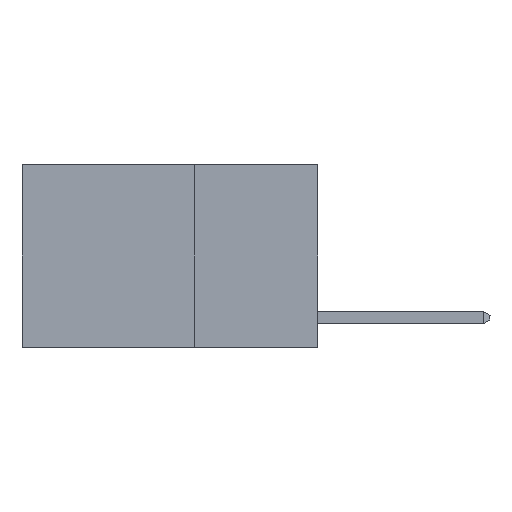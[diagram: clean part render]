
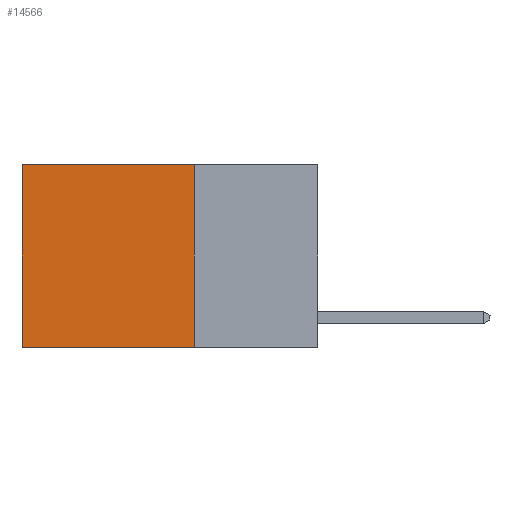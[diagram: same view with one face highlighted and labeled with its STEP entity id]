
A CAD part, left-side view. The second image highlights one B-rep face of the part: STEP entity #14566.
In plain terms, the highlighted planar face has unit normal (-1, 0, 0).
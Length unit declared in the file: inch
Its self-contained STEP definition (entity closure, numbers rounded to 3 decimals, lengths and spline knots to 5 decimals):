
#172 = VERTEX_POINT ( 'NONE', #23151 ) ;
#350 = CARTESIAN_POINT ( 'NONE',  ( 0.2625, 0.6, 0. ) ) ;
#618 = DIRECTION ( 'NONE',  ( 0., 1., 0. ) ) ;
#1610 = EDGE_CURVE ( 'NONE', #24879, #21335, #2845, .T. ) ;
#2148 = ORIENTED_EDGE ( 'NONE', *, *, #1610, .T. ) ;
#2246 = EDGE_CURVE ( 'NONE', #24879, #19010, #6435, .T. ) ;
#2845 = LINE ( 'NONE', #22204, #20345 ) ;
#4067 = EDGE_LOOP ( 'NONE', ( #6890, #4410, #8324, #2148 ) ) ;
#4410 = ORIENTED_EDGE ( 'NONE', *, *, #4507, .F. ) ;
#4507 = EDGE_CURVE ( 'NONE', #19010, #172, #23242, .T. ) ;
#5208 = DIRECTION ( 'NONE',  ( 0., 0., -1. ) ) ;
#6435 = LINE ( 'NONE', #7169, #16072 ) ;
#6767 = DIRECTION ( 'NONE',  ( 0., 1., 0. ) ) ;
#6890 = ORIENTED_EDGE ( 'NONE', *, *, #19597, .T. ) ;
#7169 = CARTESIAN_POINT ( 'NONE',  ( 0.2625, 0.25, 0. ) ) ;
#8324 = ORIENTED_EDGE ( 'NONE', *, *, #2246, .F. ) ;
#9020 = VECTOR ( 'NONE', #618, 39.37008 ) ;
#9143 = CARTESIAN_POINT ( 'NONE',  ( 0.2625, 0.25, 0. ) ) ;
#10272 = CARTESIAN_POINT ( 'NONE',  ( 0.2625, 0.25, -0.37 ) ) ;
#10679 = CARTESIAN_POINT ( 'NONE',  ( 0.2625, 0.6, 0. ) ) ;
#11058 = DIRECTION ( 'NONE',  ( 1., 0., 0. ) ) ;
#13156 = LINE ( 'NONE', #350, #23472 ) ;
#14566 = ADVANCED_FACE ( 'NONE', ( #23592 ), #20686, .F. ) ;
#15811 = DIRECTION ( 'NONE',  ( 0., 0., -1. ) ) ;
#16072 = VECTOR ( 'NONE', #5208, 39.37008 ) ;
#16746 = CARTESIAN_POINT ( 'NONE',  ( 0.2625, 0.25, 0. ) ) ;
#17666 = AXIS2_PLACEMENT_3D ( 'NONE', #9143, #11058, #24646 ) ;
#19010 = VERTEX_POINT ( 'NONE', #10272 ) ;
#19597 = EDGE_CURVE ( 'NONE', #21335, #172, #13156, .T. ) ;
#20345 = VECTOR ( 'NONE', #6767, 39.37008 ) ;
#20686 = PLANE ( 'NONE',  #17666 ) ;
#21335 = VERTEX_POINT ( 'NONE', #10679 ) ;
#22204 = CARTESIAN_POINT ( 'NONE',  ( 0.2625, 0.25, 0. ) ) ;
#23151 = CARTESIAN_POINT ( 'NONE',  ( 0.2625, 0.6, -0.37 ) ) ;
#23242 = LINE ( 'NONE', #23827, #9020 ) ;
#23472 = VECTOR ( 'NONE', #15811, 39.37008 ) ;
#23592 = FACE_OUTER_BOUND ( 'NONE', #4067, .T. ) ;
#23827 = CARTESIAN_POINT ( 'NONE',  ( 0.2625, 0.25, -0.37 ) ) ;
#24646 = DIRECTION ( 'NONE',  ( 0., 0., -1. ) ) ;
#24879 = VERTEX_POINT ( 'NONE', #16746 ) ;
